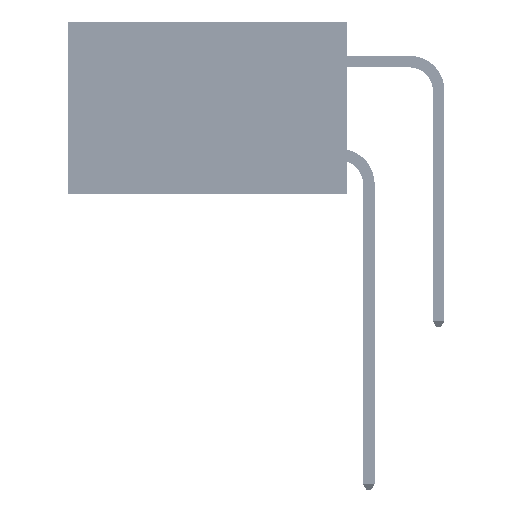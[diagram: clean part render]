
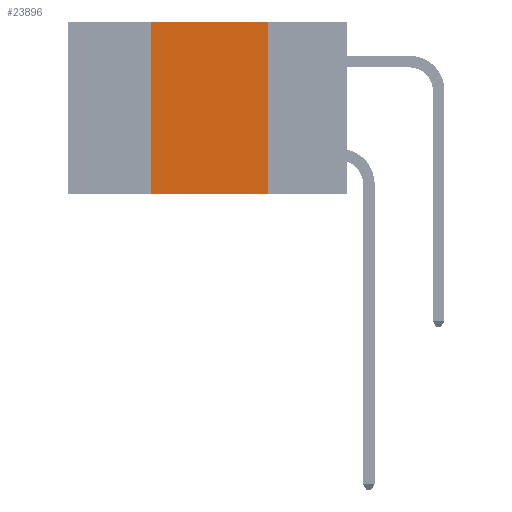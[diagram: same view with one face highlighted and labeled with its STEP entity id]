
A CAD part, left-side view. The second image highlights one B-rep face of the part: STEP entity #23896.
In plain terms, the highlighted planar face has unit normal (-1, 0, 0).
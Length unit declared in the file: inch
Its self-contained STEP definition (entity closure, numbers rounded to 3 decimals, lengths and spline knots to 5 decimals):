
#361 = ORIENTED_EDGE ( 'NONE', *, *, #13093, .F. ) ;
#1204 = CARTESIAN_POINT ( 'NONE',  ( 0., 0.6, 0. ) ) ;
#1853 = CARTESIAN_POINT ( 'NONE',  ( 0., 0.42, 0. ) ) ;
#3331 = EDGE_CURVE ( 'NONE', #35113, #48841, #35855, .T. ) ;
#3669 = CARTESIAN_POINT ( 'NONE',  ( 0., 0.42, -0.37 ) ) ;
#3962 = EDGE_CURVE ( 'NONE', #42430, #48841, #27502, .T. ) ;
#4981 = DIRECTION ( 'NONE',  ( 0., 0., -1. ) ) ;
#6074 = LINE ( 'NONE', #49087, #49371 ) ;
#8285 = DIRECTION ( 'NONE',  ( 0., 0., 1. ) ) ;
#13093 = EDGE_CURVE ( 'NONE', #31271, #42430, #19089, .T. ) ;
#13956 = VECTOR ( 'NONE', #48722, 39.37008 ) ;
#14373 = ORIENTED_EDGE ( 'NONE', *, *, #3962, .F. ) ;
#16448 = ORIENTED_EDGE ( 'NONE', *, *, #3331, .T. ) ;
#17776 = CARTESIAN_POINT ( 'NONE',  ( 0., 0.6, 0. ) ) ;
#18838 = EDGE_LOOP ( 'NONE', ( #14373, #361, #40558, #16448 ) ) ;
#19089 = LINE ( 'NONE', #17776, #41693 ) ;
#19126 = VECTOR ( 'NONE', #53334, 39.37008 ) ;
#23896 = ADVANCED_FACE ( 'NONE', ( #48884 ), #46696, .F. ) ;
#27502 = LINE ( 'NONE', #41558, #19126 ) ;
#31271 = VERTEX_POINT ( 'NONE', #1853 ) ;
#35113 = VERTEX_POINT ( 'NONE', #3669 ) ;
#35855 = LINE ( 'NONE', #40083, #13956 ) ;
#36147 = CARTESIAN_POINT ( 'NONE',  ( 0., 0.17, 0. ) ) ;
#40083 = CARTESIAN_POINT ( 'NONE',  ( 0., 0.6, -0.37 ) ) ;
#40093 = CARTESIAN_POINT ( 'NONE',  ( 0., 0.17, -0.37 ) ) ;
#40558 = ORIENTED_EDGE ( 'NONE', *, *, #49043, .F. ) ;
#41558 = CARTESIAN_POINT ( 'NONE',  ( 0., 0.17, 0. ) ) ;
#41693 = VECTOR ( 'NONE', #50221, 39.37008 ) ;
#42430 = VERTEX_POINT ( 'NONE', #36147 ) ;
#42549 = DIRECTION ( 'NONE',  ( 1., 0., 0. ) ) ;
#46696 = PLANE ( 'NONE',  #49278 ) ;
#48722 = DIRECTION ( 'NONE',  ( 0., -1., 0. ) ) ;
#48841 = VERTEX_POINT ( 'NONE', #40093 ) ;
#48884 = FACE_OUTER_BOUND ( 'NONE', #18838, .T. ) ;
#49043 = EDGE_CURVE ( 'NONE', #35113, #31271, #6074, .T. ) ;
#49087 = CARTESIAN_POINT ( 'NONE',  ( 0., 0.42, 0. ) ) ;
#49278 = AXIS2_PLACEMENT_3D ( 'NONE', #1204, #42549, #4981 ) ;
#49371 = VECTOR ( 'NONE', #8285, 39.37008 ) ;
#50221 = DIRECTION ( 'NONE',  ( 0., -1., 0. ) ) ;
#53334 = DIRECTION ( 'NONE',  ( 0., 0., -1. ) ) ;
